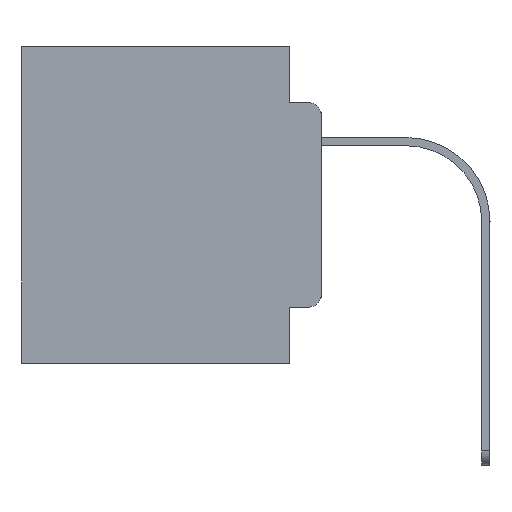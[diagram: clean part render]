
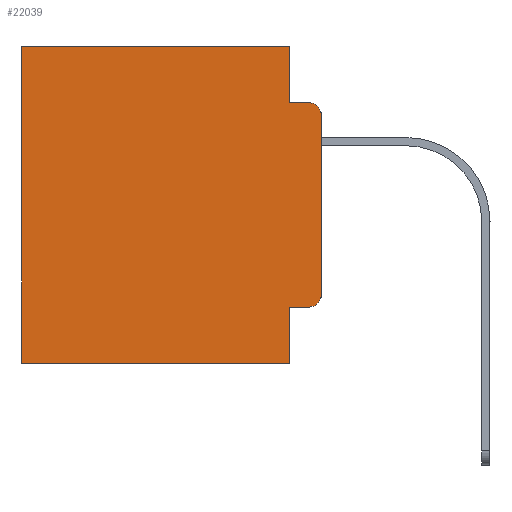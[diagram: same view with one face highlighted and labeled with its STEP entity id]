
A CAD part, left-side view. The second image highlights one B-rep face of the part: STEP entity #22039.
In plain terms, the highlighted planar face has unit normal (-1, 0, 0).
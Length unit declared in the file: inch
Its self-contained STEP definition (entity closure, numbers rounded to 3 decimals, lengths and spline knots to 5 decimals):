
#213 = CARTESIAN_POINT ( 'NONE',  ( 0.298, 0.051, -0.0885 ) ) ;
#277 = ORIENTED_EDGE ( 'NONE', *, *, #18089, .T. ) ;
#412 = DIRECTION ( 'NONE',  ( 0., 0., -1. ) ) ;
#575 = FACE_OUTER_BOUND ( 'NONE', #8127, .T. ) ;
#872 = DIRECTION ( 'NONE',  ( 0., 0., -1. ) ) ;
#1035 = LINE ( 'NONE', #12162, #18707 ) ;
#1452 = CARTESIAN_POINT ( 'NONE',  ( 0.298, 0.02, -0.0885 ) ) ;
#1459 = ORIENTED_EDGE ( 'NONE', *, *, #20834, .T. ) ;
#1582 = CARTESIAN_POINT ( 'NONE',  ( 0.298, 0.051, 0. ) ) ;
#1604 = LINE ( 'NONE', #9915, #10378 ) ;
#1927 = VERTEX_POINT ( 'NONE', #1582 ) ;
#1937 = CARTESIAN_POINT ( 'NONE',  ( 0.298, 0., 0. ) ) ;
#2007 = EDGE_CURVE ( 'NONE', #20739, #2832, #21243, .T. ) ;
#2058 = DIRECTION ( 'NONE',  ( 0., 1., 0. ) ) ;
#2832 = VERTEX_POINT ( 'NONE', #1452 ) ;
#3181 = VERTEX_POINT ( 'NONE', #4295 ) ;
#3443 = CARTESIAN_POINT ( 'NONE',  ( 0.298, 0., -0.1085 ) ) ;
#4295 = CARTESIAN_POINT ( 'NONE',  ( 0.298, 0.02, -0.4115 ) ) ;
#4307 = VECTOR ( 'NONE', #412, 39.37008 ) ;
#4428 = VECTOR ( 'NONE', #872, 39.37008 ) ;
#4692 = LINE ( 'NONE', #23431, #4428 ) ;
#4921 = CARTESIAN_POINT ( 'NONE',  ( 0.298, 0.473, 0. ) ) ;
#5113 = DIRECTION ( 'NONE',  ( 0., 0., -1. ) ) ;
#5886 = LINE ( 'NONE', #1937, #21862 ) ;
#6038 = LINE ( 'NONE', #6181, #15749 ) ;
#6181 = CARTESIAN_POINT ( 'NONE',  ( 0.298, 0., -0.5 ) ) ;
#6204 = EDGE_CURVE ( 'NONE', #6730, #2832, #11162, .T. ) ;
#6730 = VERTEX_POINT ( 'NONE', #3443 ) ;
#7322 = CARTESIAN_POINT ( 'NONE',  ( 0.298, 0.051, -0.4115 ) ) ;
#7912 = VECTOR ( 'NONE', #23443, 39.37008 ) ;
#7918 = CARTESIAN_POINT ( 'NONE',  ( 0.298, 0.051, -0.0885 ) ) ;
#8127 = EDGE_LOOP ( 'NONE', ( #18531, #9961, #16458, #11089, #277, #1459, #23891, #9950, #16139, #17078 ) ) ;
#8262 = EDGE_CURVE ( 'NONE', #3181, #12636, #9914, .T. ) ;
#8582 = PLANE ( 'NONE',  #23158 ) ;
#8666 = DIRECTION ( 'NONE',  ( 0., 0., -1. ) ) ;
#8865 = DIRECTION ( 'NONE',  ( 0., 0., -1. ) ) ;
#9914 = CIRCLE ( 'NONE', #26103, 0.02 ) ;
#9915 = CARTESIAN_POINT ( 'NONE',  ( 0.298, 0.051, 0. ) ) ;
#9950 = ORIENTED_EDGE ( 'NONE', *, *, #14474, .F. ) ;
#9961 = ORIENTED_EDGE ( 'NONE', *, *, #6204, .T. ) ;
#10298 = EDGE_CURVE ( 'NONE', #23224, #21369, #6038, .T. ) ;
#10378 = VECTOR ( 'NONE', #24193, 39.37008 ) ;
#10772 = DIRECTION ( 'NONE',  ( 1., 0., 0. ) ) ;
#11089 = ORIENTED_EDGE ( 'NONE', *, *, #16200, .F. ) ;
#11126 = CARTESIAN_POINT ( 'NONE',  ( 0.298, 0.02, -0.1085 ) ) ;
#11162 = CIRCLE ( 'NONE', #14624, 0.02 ) ;
#11277 = VERTEX_POINT ( 'NONE', #11472 ) ;
#11472 = CARTESIAN_POINT ( 'NONE',  ( 0.298, 0.473, 0. ) ) ;
#12162 = CARTESIAN_POINT ( 'NONE',  ( 0.298, 0.051, 0. ) ) ;
#12636 = VERTEX_POINT ( 'NONE', #26134 ) ;
#13170 = DIRECTION ( 'NONE',  ( -1., 0., 0. ) ) ;
#13357 = LINE ( 'NONE', #15438, #26115 ) ;
#13729 = CARTESIAN_POINT ( 'NONE',  ( 0.298, 0.473, -0.5 ) ) ;
#14474 = EDGE_CURVE ( 'NONE', #18200, #23224, #1604, .T. ) ;
#14624 = AXIS2_PLACEMENT_3D ( 'NONE', #11126, #13170, #17574 ) ;
#15285 = EDGE_CURVE ( 'NONE', #18200, #3181, #13357, .T. ) ;
#15438 = CARTESIAN_POINT ( 'NONE',  ( 0.298, 0.051, -0.4115 ) ) ;
#15749 = VECTOR ( 'NONE', #18622, 39.37008 ) ;
#16139 = ORIENTED_EDGE ( 'NONE', *, *, #15285, .T. ) ;
#16200 = EDGE_CURVE ( 'NONE', #1927, #20739, #1035, .T. ) ;
#16458 = ORIENTED_EDGE ( 'NONE', *, *, #2007, .F. ) ;
#17078 = ORIENTED_EDGE ( 'NONE', *, *, #8262, .T. ) ;
#17574 = DIRECTION ( 'NONE',  ( 0., 0., -1. ) ) ;
#18089 = EDGE_CURVE ( 'NONE', #1927, #11277, #5886, .T. ) ;
#18200 = VERTEX_POINT ( 'NONE', #7322 ) ;
#18531 = ORIENTED_EDGE ( 'NONE', *, *, #23652, .F. ) ;
#18622 = DIRECTION ( 'NONE',  ( 0., 1., 0. ) ) ;
#18707 = VECTOR ( 'NONE', #5113, 39.37008 ) ;
#19131 = LINE ( 'NONE', #4921, #4307 ) ;
#20739 = VERTEX_POINT ( 'NONE', #7918 ) ;
#20834 = EDGE_CURVE ( 'NONE', #11277, #21369, #19131, .T. ) ;
#21243 = LINE ( 'NONE', #213, #7912 ) ;
#21369 = VERTEX_POINT ( 'NONE', #13729 ) ;
#21465 = CARTESIAN_POINT ( 'NONE',  ( 0.298, 0., 0. ) ) ;
#21620 = CARTESIAN_POINT ( 'NONE',  ( 0.298, 0.051, -0.5 ) ) ;
#21683 = DIRECTION ( 'NONE',  ( -1., 0., 0. ) ) ;
#21862 = VECTOR ( 'NONE', #2058, 39.37008 ) ;
#22039 = ADVANCED_FACE ( 'NONE', ( #575 ), #8582, .F. ) ;
#23158 = AXIS2_PLACEMENT_3D ( 'NONE', #21465, #10772, #8865 ) ;
#23224 = VERTEX_POINT ( 'NONE', #21620 ) ;
#23431 = CARTESIAN_POINT ( 'NONE',  ( 0.298, 0., 0. ) ) ;
#23443 = DIRECTION ( 'NONE',  ( 0., -1., 0. ) ) ;
#23652 = EDGE_CURVE ( 'NONE', #6730, #12636, #4692, .T. ) ;
#23756 = CARTESIAN_POINT ( 'NONE',  ( 0.298, 0.02, -0.3915 ) ) ;
#23803 = DIRECTION ( 'NONE',  ( 0., -1., 0. ) ) ;
#23891 = ORIENTED_EDGE ( 'NONE', *, *, #10298, .F. ) ;
#24193 = DIRECTION ( 'NONE',  ( 0., 0., -1. ) ) ;
#26103 = AXIS2_PLACEMENT_3D ( 'NONE', #23756, #21683, #8666 ) ;
#26115 = VECTOR ( 'NONE', #23803, 39.37008 ) ;
#26134 = CARTESIAN_POINT ( 'NONE',  ( 0.298, 0., -0.3915 ) ) ;
